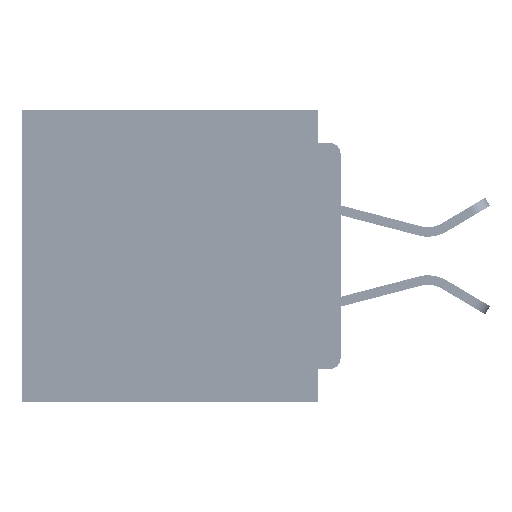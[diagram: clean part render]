
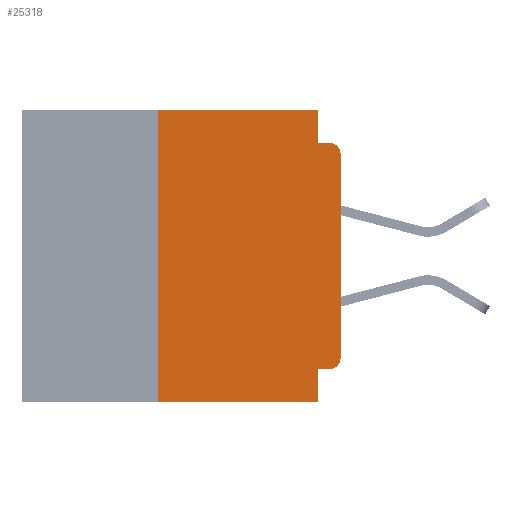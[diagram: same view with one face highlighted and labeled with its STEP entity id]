
A CAD part, left-side view. The second image highlights one B-rep face of the part: STEP entity #25318.
In plain terms, the highlighted planar face has unit normal (-1, 0, 0).
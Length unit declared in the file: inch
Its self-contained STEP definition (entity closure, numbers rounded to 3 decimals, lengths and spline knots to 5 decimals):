
#239 = DIRECTION ( 'NONE',  ( 0., -1., 0. ) ) ;
#331 = DIRECTION ( 'NONE',  ( 0., -1., 0. ) ) ;
#1033 = VECTOR ( 'NONE', #239, 39.37008 ) ;
#1081 = EDGE_CURVE ( 'NONE', #10819, #10590, #34764, .T. ) ;
#1387 = AXIS2_PLACEMENT_3D ( 'NONE', #15636, #47016, #20218 ) ;
#1730 = CARTESIAN_POINT ( 'NONE',  ( 0., 0., -0.045 ) ) ;
#3450 = EDGE_CURVE ( 'NONE', #8106, #10819, #50524, .T. ) ;
#4131 = DIRECTION ( 'NONE',  ( 0., 0., -1. ) ) ;
#6686 = CARTESIAN_POINT ( 'NONE',  ( 0., 0., 0. ) ) ;
#7778 = VERTEX_POINT ( 'NONE', #30502 ) ;
#8106 = VERTEX_POINT ( 'NONE', #14547 ) ;
#8162 = VECTOR ( 'NONE', #42651, 39.37008 ) ;
#8291 = ORIENTED_EDGE ( 'NONE', *, *, #42058, .F. ) ;
#8819 = CARTESIAN_POINT ( 'NONE',  ( 0., 0., -0.06 ) ) ;
#10494 = ORIENTED_EDGE ( 'NONE', *, *, #57971, .T. ) ;
#10590 = VERTEX_POINT ( 'NONE', #46532 ) ;
#10819 = VERTEX_POINT ( 'NONE', #53535 ) ;
#11055 = VECTOR ( 'NONE', #27018, 39.37008 ) ;
#11311 = PLANE ( 'NONE',  #55117 ) ;
#13029 = LINE ( 'NONE', #26997, #1033 ) ;
#14547 = CARTESIAN_POINT ( 'NONE',  ( 0., 0.031, 0. ) ) ;
#15552 = ORIENTED_EDGE ( 'NONE', *, *, #46444, .T. ) ;
#15636 = CARTESIAN_POINT ( 'NONE',  ( 0., 0.015, -0.06 ) ) ;
#17187 = DIRECTION ( 'NONE',  ( 0., 1., 0. ) ) ;
#17188 = EDGE_CURVE ( 'NONE', #18473, #21661, #35416, .T. ) ;
#17930 = ORIENTED_EDGE ( 'NONE', *, *, #34380, .T. ) ;
#18405 = LINE ( 'NONE', #50707, #39502 ) ;
#18473 = VERTEX_POINT ( 'NONE', #57733 ) ;
#18719 = ORIENTED_EDGE ( 'NONE', *, *, #17188, .F. ) ;
#18970 = CIRCLE ( 'NONE', #47580, 0.015 ) ;
#19894 = VECTOR ( 'NONE', #17187, 39.37008 ) ;
#20150 = LINE ( 'NONE', #6686, #8162 ) ;
#20218 = DIRECTION ( 'NONE',  ( 0., 0., -1. ) ) ;
#20377 = CARTESIAN_POINT ( 'NONE',  ( 0., 0.437, 0. ) ) ;
#21579 = CARTESIAN_POINT ( 'NONE',  ( 0., 0.031, 0. ) ) ;
#21661 = VERTEX_POINT ( 'NONE', #31261 ) ;
#22084 = VECTOR ( 'NONE', #4131, 39.37008 ) ;
#23027 = LINE ( 'NONE', #31307, #11055 ) ;
#23035 = DIRECTION ( 'NONE',  ( -1., 0., 0. ) ) ;
#24891 = DIRECTION ( 'NONE',  ( 0., 0., -1. ) ) ;
#25318 = ADVANCED_FACE ( 'NONE', ( #50916 ), #11311, .F. ) ;
#25618 = EDGE_CURVE ( 'NONE', #30847, #8106, #13029, .T. ) ;
#26571 = CARTESIAN_POINT ( 'NONE',  ( 0., 0.031, -0.4 ) ) ;
#26997 = CARTESIAN_POINT ( 'NONE',  ( 0., 0.437, 0. ) ) ;
#27018 = DIRECTION ( 'NONE',  ( 0., 0., 1. ) ) ;
#28980 = LINE ( 'NONE', #35108, #19894 ) ;
#29994 = CARTESIAN_POINT ( 'NONE',  ( 0., 0.015, -0.355 ) ) ;
#30502 = CARTESIAN_POINT ( 'NONE',  ( 0., 0.25, -0.4 ) ) ;
#30691 = VERTEX_POINT ( 'NONE', #49840 ) ;
#30847 = VERTEX_POINT ( 'NONE', #42112 ) ;
#31241 = CIRCLE ( 'NONE', #1387, 0.015 ) ;
#31261 = CARTESIAN_POINT ( 'NONE',  ( 0., 0.031, -0.4 ) ) ;
#31307 = CARTESIAN_POINT ( 'NONE',  ( 0., 0.25, -0.4 ) ) ;
#32961 = DIRECTION ( 'NONE',  ( 0., -1., 0. ) ) ;
#34380 = EDGE_CURVE ( 'NONE', #30691, #45533, #20150, .T. ) ;
#34764 = LINE ( 'NONE', #1730, #45208 ) ;
#35108 = CARTESIAN_POINT ( 'NONE',  ( 0., 0., -0.355 ) ) ;
#35269 = ORIENTED_EDGE ( 'NONE', *, *, #37358, .F. ) ;
#35416 = LINE ( 'NONE', #26571, #22084 ) ;
#37358 = EDGE_CURVE ( 'NONE', #44049, #18473, #28980, .T. ) ;
#39502 = VECTOR ( 'NONE', #32961, 39.37008 ) ;
#42058 = EDGE_CURVE ( 'NONE', #7778, #30847, #23027, .T. ) ;
#42112 = CARTESIAN_POINT ( 'NONE',  ( 0., 0.25, 0. ) ) ;
#42651 = DIRECTION ( 'NONE',  ( 0., 0., 1. ) ) ;
#42866 = ORIENTED_EDGE ( 'NONE', *, *, #1081, .F. ) ;
#44049 = VERTEX_POINT ( 'NONE', #29994 ) ;
#44445 = ORIENTED_EDGE ( 'NONE', *, *, #50941, .T. ) ;
#45208 = VECTOR ( 'NONE', #331, 39.37008 ) ;
#45533 = VERTEX_POINT ( 'NONE', #8819 ) ;
#46444 = EDGE_CURVE ( 'NONE', #44049, #30691, #18970, .T. ) ;
#46532 = CARTESIAN_POINT ( 'NONE',  ( 0., 0.015, -0.045 ) ) ;
#47016 = DIRECTION ( 'NONE',  ( -1., 0., 0. ) ) ;
#47580 = AXIS2_PLACEMENT_3D ( 'NONE', #49801, #23035, #54299 ) ;
#49136 = VECTOR ( 'NONE', #52856, 39.37008 ) ;
#49801 = CARTESIAN_POINT ( 'NONE',  ( 0., 0.015, -0.34 ) ) ;
#49840 = CARTESIAN_POINT ( 'NONE',  ( 0., 0., -0.34 ) ) ;
#50524 = LINE ( 'NONE', #21579, #49136 ) ;
#50707 = CARTESIAN_POINT ( 'NONE',  ( 0., 0.437, -0.4 ) ) ;
#50916 = FACE_OUTER_BOUND ( 'NONE', #55107, .T. ) ;
#50941 = EDGE_CURVE ( 'NONE', #45533, #10590, #31241, .T. ) ;
#51645 = DIRECTION ( 'NONE',  ( 1., 0., 0. ) ) ;
#52247 = ORIENTED_EDGE ( 'NONE', *, *, #25618, .F. ) ;
#52856 = DIRECTION ( 'NONE',  ( 0., 0., -1. ) ) ;
#53535 = CARTESIAN_POINT ( 'NONE',  ( 0., 0.031, -0.045 ) ) ;
#54299 = DIRECTION ( 'NONE',  ( 0., 0., -1. ) ) ;
#55107 = EDGE_LOOP ( 'NONE', ( #17930, #44445, #42866, #56723, #52247, #8291, #10494, #18719, #35269, #15552 ) ) ;
#55117 = AXIS2_PLACEMENT_3D ( 'NONE', #20377, #51645, #24891 ) ;
#56723 = ORIENTED_EDGE ( 'NONE', *, *, #3450, .F. ) ;
#57733 = CARTESIAN_POINT ( 'NONE',  ( 0., 0.031, -0.355 ) ) ;
#57971 = EDGE_CURVE ( 'NONE', #7778, #21661, #18405, .T. ) ;
